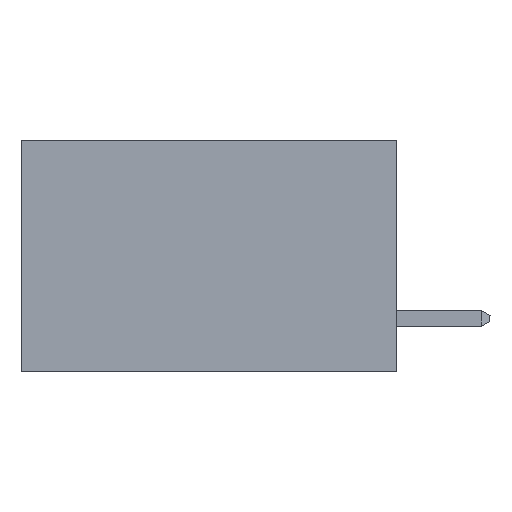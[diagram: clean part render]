
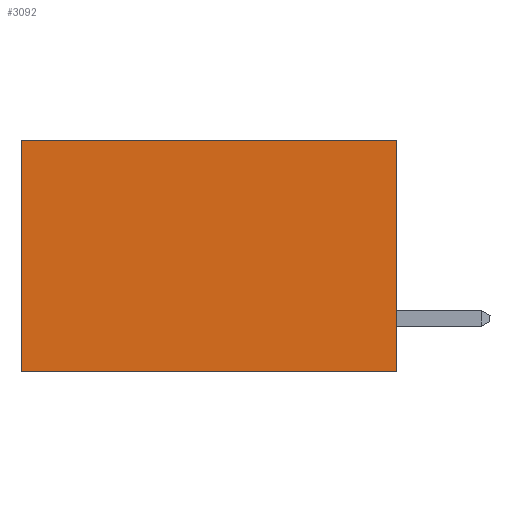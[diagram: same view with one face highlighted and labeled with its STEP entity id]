
A CAD part, left-side view. The second image highlights one B-rep face of the part: STEP entity #3092.
In plain terms, the highlighted planar face has unit normal (-1, 0, 0).
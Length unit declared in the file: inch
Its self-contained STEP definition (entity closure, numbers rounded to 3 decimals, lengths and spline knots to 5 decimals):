
#334 = CARTESIAN_POINT ( 'NONE',  ( 0.2615, 0., -0.37 ) ) ;
#607 = VERTEX_POINT ( 'NONE', #9035 ) ;
#645 = EDGE_CURVE ( 'NONE', #13067, #8998, #4584, .T. ) ;
#985 = CARTESIAN_POINT ( 'NONE',  ( 0.2615, 0.6, -0.37 ) ) ;
#1068 = CARTESIAN_POINT ( 'NONE',  ( 0.2615, 0., 0. ) ) ;
#1516 = ORIENTED_EDGE ( 'NONE', *, *, #2145, .F. ) ;
#1688 = EDGE_LOOP ( 'NONE', ( #12746, #1516, #2094, #4849 ) ) ;
#2094 = ORIENTED_EDGE ( 'NONE', *, *, #645, .F. ) ;
#2145 = EDGE_CURVE ( 'NONE', #8998, #607, #4342, .T. ) ;
#2376 = DIRECTION ( 'NONE',  ( 0., 0., -1. ) ) ;
#2660 = LINE ( 'NONE', #1068, #9286 ) ;
#3092 = ADVANCED_FACE ( 'NONE', ( #4304 ), #11766, .F. ) ;
#3946 = CARTESIAN_POINT ( 'NONE',  ( 0.2615, 0., -0.37 ) ) ;
#4304 = FACE_OUTER_BOUND ( 'NONE', #1688, .T. ) ;
#4342 = LINE ( 'NONE', #334, #10493 ) ;
#4584 = LINE ( 'NONE', #3946, #7433 ) ;
#4730 = CARTESIAN_POINT ( 'NONE',  ( 0.2615, 0., 0. ) ) ;
#4786 = VECTOR ( 'NONE', #10868, 39.37008 ) ;
#4849 = ORIENTED_EDGE ( 'NONE', *, *, #9271, .T. ) ;
#5052 = DIRECTION ( 'NONE',  ( 0., 1., 0. ) ) ;
#5513 = CARTESIAN_POINT ( 'NONE',  ( 0.2615, 0., -0.37 ) ) ;
#7196 = AXIS2_PLACEMENT_3D ( 'NONE', #5513, #7532, #7687 ) ;
#7433 = VECTOR ( 'NONE', #2376, 39.37008 ) ;
#7532 = DIRECTION ( 'NONE',  ( 1., 0., 0. ) ) ;
#7687 = DIRECTION ( 'NONE',  ( 0., 0., -1. ) ) ;
#7868 = CARTESIAN_POINT ( 'NONE',  ( 0.2615, 0., -0.37 ) ) ;
#8467 = DIRECTION ( 'NONE',  ( 0., 1., 0. ) ) ;
#8998 = VERTEX_POINT ( 'NONE', #7868 ) ;
#9035 = CARTESIAN_POINT ( 'NONE',  ( 0.2615, 0.6, -0.37 ) ) ;
#9271 = EDGE_CURVE ( 'NONE', #13067, #12319, #2660, .T. ) ;
#9286 = VECTOR ( 'NONE', #8467, 39.37008 ) ;
#10493 = VECTOR ( 'NONE', #5052, 39.37008 ) ;
#10868 = DIRECTION ( 'NONE',  ( 0., 0., -1. ) ) ;
#11352 = LINE ( 'NONE', #985, #4786 ) ;
#11766 = PLANE ( 'NONE',  #7196 ) ;
#11856 = CARTESIAN_POINT ( 'NONE',  ( 0.2615, 0.6, 0. ) ) ;
#12319 = VERTEX_POINT ( 'NONE', #11856 ) ;
#12746 = ORIENTED_EDGE ( 'NONE', *, *, #13428, .T. ) ;
#13067 = VERTEX_POINT ( 'NONE', #4730 ) ;
#13428 = EDGE_CURVE ( 'NONE', #12319, #607, #11352, .T. ) ;
